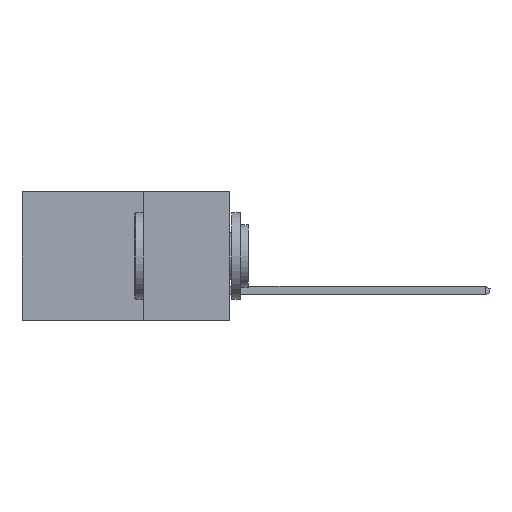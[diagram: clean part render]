
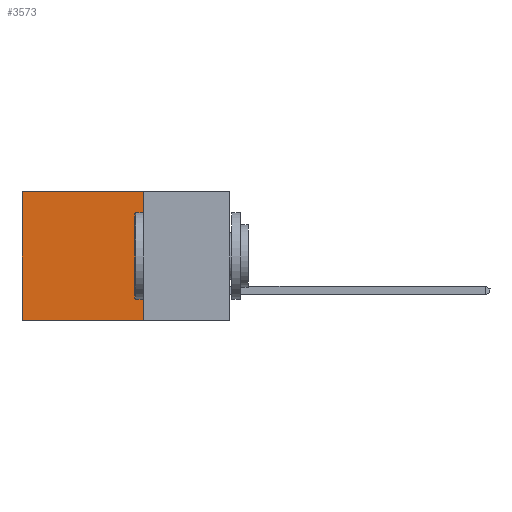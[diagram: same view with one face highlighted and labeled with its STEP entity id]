
A CAD part, left-side view. The second image highlights one B-rep face of the part: STEP entity #3573.
In plain terms, the highlighted planar face has unit normal (-1, 0, 0).
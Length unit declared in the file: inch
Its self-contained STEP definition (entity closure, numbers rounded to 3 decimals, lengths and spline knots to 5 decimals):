
#18 = VERTEX_POINT ( 'NONE', #10252 ) ;
#219 = EDGE_CURVE ( 'NONE', #13085, #6737, #11067, .T. ) ;
#407 = DIRECTION ( 'NONE',  ( 0., 1., 0. ) ) ;
#451 = VECTOR ( 'NONE', #13676, 39.37008 ) ;
#878 = LINE ( 'NONE', #2007, #451 ) ;
#1159 = DIRECTION ( 'NONE',  ( 0., 1., 0. ) ) ;
#1735 = EDGE_CURVE ( 'NONE', #16504, #18, #15918, .T. ) ;
#1898 = EDGE_CURVE ( 'NONE', #16504, #13085, #878, .T. ) ;
#1938 = VECTOR ( 'NONE', #407, 39.37008 ) ;
#2007 = CARTESIAN_POINT ( 'NONE',  ( 0.2615, 0.25, -0.37 ) ) ;
#2563 = CARTESIAN_POINT ( 'NONE',  ( 0.2615, 0.25, -0.37 ) ) ;
#2894 = VECTOR ( 'NONE', #3728, 39.37008 ) ;
#3133 = CARTESIAN_POINT ( 'NONE',  ( 0.2615, 0.25, 0. ) ) ;
#3573 = ADVANCED_FACE ( 'NONE', ( #6733 ), #11044, .F. ) ;
#3728 = DIRECTION ( 'NONE',  ( 0., 0., -1. ) ) ;
#5569 = CARTESIAN_POINT ( 'NONE',  ( 0.2615, 0.6, -0.37 ) ) ;
#6031 = VECTOR ( 'NONE', #1159, 39.37008 ) ;
#6733 = FACE_OUTER_BOUND ( 'NONE', #17527, .T. ) ;
#6737 = VERTEX_POINT ( 'NONE', #10123 ) ;
#8223 = CARTESIAN_POINT ( 'NONE',  ( 0.2615, 0.25, 0. ) ) ;
#8337 = ORIENTED_EDGE ( 'NONE', *, *, #13136, .T. ) ;
#8816 = AXIS2_PLACEMENT_3D ( 'NONE', #9642, #9559, #18300 ) ;
#8876 = ORIENTED_EDGE ( 'NONE', *, *, #219, .F. ) ;
#9559 = DIRECTION ( 'NONE',  ( 1., 0., 0. ) ) ;
#9642 = CARTESIAN_POINT ( 'NONE',  ( 0.2615, 0.25, -0.37 ) ) ;
#10049 = ORIENTED_EDGE ( 'NONE', *, *, #1735, .T. ) ;
#10123 = CARTESIAN_POINT ( 'NONE',  ( 0.2615, 0.6, -0.37 ) ) ;
#10252 = CARTESIAN_POINT ( 'NONE',  ( 0.2615, 0.6, 0. ) ) ;
#11044 = PLANE ( 'NONE',  #8816 ) ;
#11067 = LINE ( 'NONE', #2563, #6031 ) ;
#13085 = VERTEX_POINT ( 'NONE', #17447 ) ;
#13136 = EDGE_CURVE ( 'NONE', #18, #6737, #13623, .T. ) ;
#13623 = LINE ( 'NONE', #5569, #2894 ) ;
#13676 = DIRECTION ( 'NONE',  ( 0., 0., -1. ) ) ;
#14602 = ORIENTED_EDGE ( 'NONE', *, *, #1898, .F. ) ;
#15918 = LINE ( 'NONE', #3133, #1938 ) ;
#16504 = VERTEX_POINT ( 'NONE', #8223 ) ;
#17447 = CARTESIAN_POINT ( 'NONE',  ( 0.2615, 0.25, -0.37 ) ) ;
#17527 = EDGE_LOOP ( 'NONE', ( #8337, #8876, #14602, #10049 ) ) ;
#18300 = DIRECTION ( 'NONE',  ( 0., 0., -1. ) ) ;
